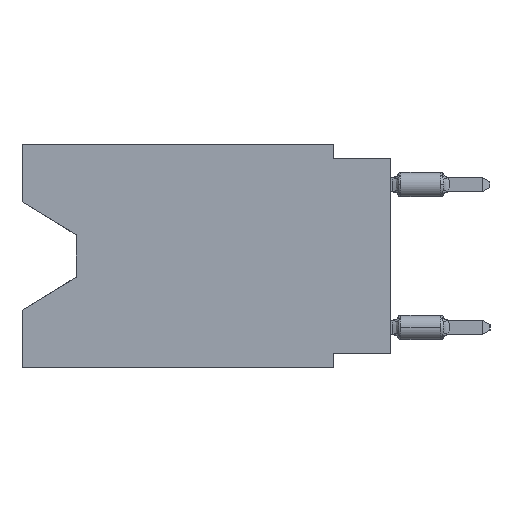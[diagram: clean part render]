
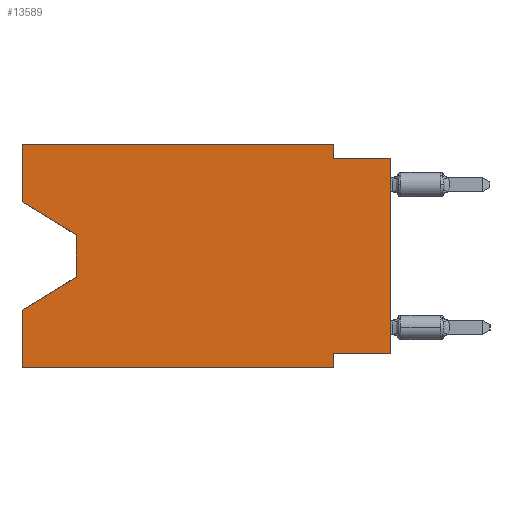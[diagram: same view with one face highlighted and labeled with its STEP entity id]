
A CAD part, left-side view. The second image highlights one B-rep face of the part: STEP entity #13589.
In plain terms, the highlighted planar face has unit normal (-1, 0, 0).
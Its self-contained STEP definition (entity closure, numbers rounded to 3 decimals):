
#168 = ORIENTED_EDGE ( 'NONE', *, *, #25486, .F. ) ;
#348 = ORIENTED_EDGE ( 'NONE', *, *, #16304, .F. ) ;
#498 = ORIENTED_EDGE ( 'NONE', *, *, #18960, .T. ) ;
#637 = VECTOR ( 'NONE', #19490, 1000. ) ;
#685 = LINE ( 'NONE', #2379, #10147 ) ;
#713 = CARTESIAN_POINT ( 'NONE',  ( 0., 0., -0.635 ) ) ;
#806 = VERTEX_POINT ( 'NONE', #4618 ) ;
#1128 = AXIS2_PLACEMENT_3D ( 'NONE', #19245, #17778, #15838 ) ;
#1286 = LINE ( 'NONE', #22896, #17644 ) ;
#1783 = ORIENTED_EDGE ( 'NONE', *, *, #11221, .T. ) ;
#2074 = CARTESIAN_POINT ( 'NONE',  ( 0., 13.97, -4.013 ) ) ;
#2379 = CARTESIAN_POINT ( 'NONE',  ( 0., 16.383, 0. ) ) ;
#2570 = EDGE_LOOP ( 'NONE', ( #14988, #498, #17324, #10502, #20628, #5032, #6494, #1783, #12864, #348, #3517, #168 ) ) ;
#2722 = VERTEX_POINT ( 'NONE', #713 ) ;
#3023 = LINE ( 'NONE', #14956, #17607 ) ;
#3072 = EDGE_CURVE ( 'NONE', #3237, #6236, #685, .T. ) ;
#3075 = VECTOR ( 'NONE', #7878, 1000. ) ;
#3237 = VERTEX_POINT ( 'NONE', #8977 ) ;
#3243 = LINE ( 'NONE', #15169, #20177 ) ;
#3476 = EDGE_CURVE ( 'NONE', #20193, #2722, #8771, .T. ) ;
#3517 = ORIENTED_EDGE ( 'NONE', *, *, #3072, .F. ) ;
#3841 = CARTESIAN_POINT ( 'NONE',  ( 0., 16.383, 0. ) ) ;
#4277 = CARTESIAN_POINT ( 'NONE',  ( 0., 0., -9.271 ) ) ;
#4300 = VERTEX_POINT ( 'NONE', #4277 ) ;
#4618 = CARTESIAN_POINT ( 'NONE',  ( 0., 2.54, -9.271 ) ) ;
#4754 = VECTOR ( 'NONE', #11749, 1000. ) ;
#4891 = DIRECTION ( 'NONE',  ( 0., -1., 0. ) ) ;
#5032 = ORIENTED_EDGE ( 'NONE', *, *, #23806, .F. ) ;
#5166 = DIRECTION ( 'NONE',  ( 0., 0., -1. ) ) ;
#5650 = LINE ( 'NONE', #10164, #13605 ) ;
#6186 = LINE ( 'NONE', #15791, #3075 ) ;
#6236 = VERTEX_POINT ( 'NONE', #12935 ) ;
#6494 = ORIENTED_EDGE ( 'NONE', *, *, #18210, .F. ) ;
#7027 = DIRECTION ( 'NONE',  ( 0., 1., 0. ) ) ;
#7171 = CARTESIAN_POINT ( 'NONE',  ( 0., 16.383, -2.546 ) ) ;
#7454 = CARTESIAN_POINT ( 'NONE',  ( 0., 0., 0. ) ) ;
#7791 = VECTOR ( 'NONE', #21341, 1000. ) ;
#7878 = DIRECTION ( 'NONE',  ( 0., 0.855, -0.519 ) ) ;
#7996 = CARTESIAN_POINT ( 'NONE',  ( 0., 16.383, -7.36 ) ) ;
#8167 = EDGE_CURVE ( 'NONE', #12371, #8222, #6186, .T. ) ;
#8222 = VERTEX_POINT ( 'NONE', #7996 ) ;
#8249 = VECTOR ( 'NONE', #4891, 1000. ) ;
#8425 = CARTESIAN_POINT ( 'NONE',  ( 0., 16.383, -9.906 ) ) ;
#8771 = LINE ( 'NONE', #22625, #8249 ) ;
#8953 = CARTESIAN_POINT ( 'NONE',  ( 0., 2.54, -0.635 ) ) ;
#8977 = CARTESIAN_POINT ( 'NONE',  ( 0., 16.383, 0. ) ) ;
#9430 = VECTOR ( 'NONE', #18540, 1000. ) ;
#9969 = VERTEX_POINT ( 'NONE', #7171 ) ;
#10147 = VECTOR ( 'NONE', #10657, 1000. ) ;
#10164 = CARTESIAN_POINT ( 'NONE',  ( 0., 16.383, 0. ) ) ;
#10403 = VECTOR ( 'NONE', #17866, 1000. ) ;
#10502 = ORIENTED_EDGE ( 'NONE', *, *, #10835, .F. ) ;
#10657 = DIRECTION ( 'NONE',  ( 0., -1., 0. ) ) ;
#10835 = EDGE_CURVE ( 'NONE', #14412, #8222, #21576, .T. ) ;
#11221 = EDGE_CURVE ( 'NONE', #4300, #2722, #17302, .T. ) ;
#11749 = DIRECTION ( 'NONE',  ( 0., 0., 1. ) ) ;
#12299 = LINE ( 'NONE', #2074, #10403 ) ;
#12371 = VERTEX_POINT ( 'NONE', #19716 ) ;
#12864 = ORIENTED_EDGE ( 'NONE', *, *, #3476, .F. ) ;
#12935 = CARTESIAN_POINT ( 'NONE',  ( 0., 2.54, 0. ) ) ;
#13589 = ADVANCED_FACE ( 'NONE', ( #17174 ), #13767, .F. ) ;
#13605 = VECTOR ( 'NONE', #15878, 1000. ) ;
#13767 = PLANE ( 'NONE',  #1128 ) ;
#13796 = EDGE_CURVE ( 'NONE', #14412, #14383, #14024, .T. ) ;
#14024 = LINE ( 'NONE', #8425, #9430 ) ;
#14383 = VERTEX_POINT ( 'NONE', #16689 ) ;
#14412 = VERTEX_POINT ( 'NONE', #22501 ) ;
#14956 = CARTESIAN_POINT ( 'NONE',  ( 0., 0., -9.271 ) ) ;
#14988 = ORIENTED_EDGE ( 'NONE', *, *, #24935, .T. ) ;
#15169 = CARTESIAN_POINT ( 'NONE',  ( 0., 16.383, -2.546 ) ) ;
#15769 = CARTESIAN_POINT ( 'NONE',  ( 0., 2.54, 0. ) ) ;
#15791 = CARTESIAN_POINT ( 'NONE',  ( 0., 13.97, -5.893 ) ) ;
#15838 = DIRECTION ( 'NONE',  ( 0., 0., -1. ) ) ;
#15878 = DIRECTION ( 'NONE',  ( 0., 0., 1. ) ) ;
#16304 = EDGE_CURVE ( 'NONE', #6236, #20193, #17206, .T. ) ;
#16689 = CARTESIAN_POINT ( 'NONE',  ( 0., 2.54, -9.906 ) ) ;
#17174 = FACE_OUTER_BOUND ( 'NONE', #2570, .T. ) ;
#17206 = LINE ( 'NONE', #15769, #7791 ) ;
#17302 = LINE ( 'NONE', #7454, #637 ) ;
#17324 = ORIENTED_EDGE ( 'NONE', *, *, #8167, .T. ) ;
#17607 = VECTOR ( 'NONE', #7027, 1000. ) ;
#17644 = VECTOR ( 'NONE', #5166, 1000. ) ;
#17778 = DIRECTION ( 'NONE',  ( 1., 0., 0. ) ) ;
#17866 = DIRECTION ( 'NONE',  ( 0., 0., -1. ) ) ;
#18210 = EDGE_CURVE ( 'NONE', #4300, #806, #3023, .T. ) ;
#18412 = VERTEX_POINT ( 'NONE', #21532 ) ;
#18540 = DIRECTION ( 'NONE',  ( 0., -1., 0. ) ) ;
#18960 = EDGE_CURVE ( 'NONE', #18412, #12371, #12299, .T. ) ;
#19245 = CARTESIAN_POINT ( 'NONE',  ( 0., 16.383, 0. ) ) ;
#19490 = DIRECTION ( 'NONE',  ( 0., 0., 1. ) ) ;
#19716 = CARTESIAN_POINT ( 'NONE',  ( 0., 13.97, -5.893 ) ) ;
#20177 = VECTOR ( 'NONE', #21364, 1000. ) ;
#20193 = VERTEX_POINT ( 'NONE', #8953 ) ;
#20628 = ORIENTED_EDGE ( 'NONE', *, *, #13796, .T. ) ;
#21341 = DIRECTION ( 'NONE',  ( 0., 0., -1. ) ) ;
#21364 = DIRECTION ( 'NONE',  ( 0., -0.855, -0.519 ) ) ;
#21532 = CARTESIAN_POINT ( 'NONE',  ( 0., 13.97, -4.013 ) ) ;
#21576 = LINE ( 'NONE', #3841, #4754 ) ;
#22501 = CARTESIAN_POINT ( 'NONE',  ( 0., 16.383, -9.906 ) ) ;
#22625 = CARTESIAN_POINT ( 'NONE',  ( 0., 0., -0.635 ) ) ;
#22896 = CARTESIAN_POINT ( 'NONE',  ( 0., 2.54, -9.906 ) ) ;
#23806 = EDGE_CURVE ( 'NONE', #806, #14383, #1286, .T. ) ;
#24935 = EDGE_CURVE ( 'NONE', #9969, #18412, #3243, .T. ) ;
#25486 = EDGE_CURVE ( 'NONE', #9969, #3237, #5650, .T. ) ;
